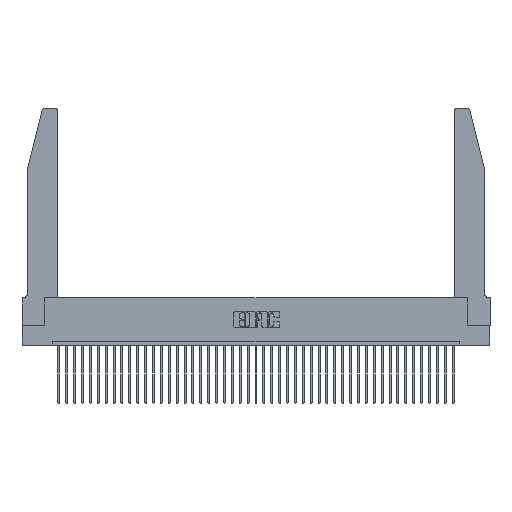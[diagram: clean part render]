
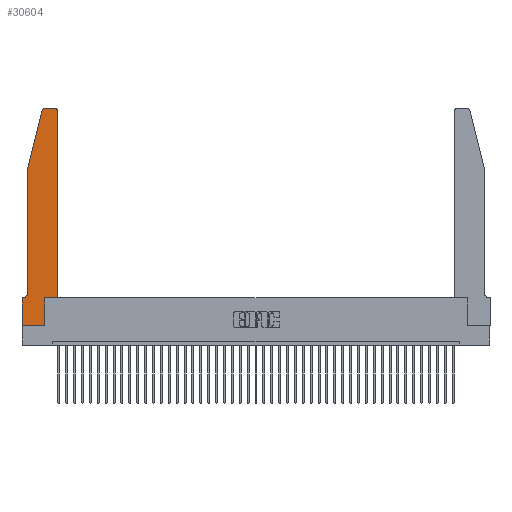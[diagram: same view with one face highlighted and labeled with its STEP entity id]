
A CAD part, top view. The second image highlights one B-rep face of the part: STEP entity #30604.
In plain terms, the highlighted planar face has unit normal (0, 0, 1).
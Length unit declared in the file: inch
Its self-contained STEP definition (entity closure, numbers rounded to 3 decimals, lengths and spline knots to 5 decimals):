
#21 = ORIENTED_EDGE ( 'NONE', *, *, #20833, .T. ) ;
#285 = LINE ( 'NONE', #1883, #33693 ) ;
#905 = AXIS2_PLACEMENT_3D ( 'NONE', #6078, #22050, #25367 ) ;
#1460 = ORIENTED_EDGE ( 'NONE', *, *, #10855, .T. ) ;
#1763 = CARTESIAN_POINT ( 'NONE',  ( 0.0055, 0.35, 0.37 ) ) ;
#1883 = CARTESIAN_POINT ( 'NONE',  ( 0.0755, 2., 0.37 ) ) ;
#2541 = CARTESIAN_POINT ( 'NONE',  ( 0.284, 2.75, 0.37 ) ) ;
#3095 = AXIS2_PLACEMENT_3D ( 'NONE', #4685, #11182, #14152 ) ;
#3257 = LINE ( 'NONE', #5155, #26515 ) ;
#4301 = CARTESIAN_POINT ( 'NONE',  ( 0.2865, 0., 0.37 ) ) ;
#4553 = ORIENTED_EDGE ( 'NONE', *, *, #19292, .T. ) ;
#4685 = CARTESIAN_POINT ( 'NONE',  ( 0., 0.35, 0.37 ) ) ;
#5155 = CARTESIAN_POINT ( 'NONE',  ( 0.0755, 0.35, 0.37 ) ) ;
#5420 = DIRECTION ( 'NONE',  ( 0., -1., 0. ) ) ;
#5426 = ORIENTED_EDGE ( 'NONE', *, *, #34416, .T. ) ;
#5532 = CARTESIAN_POINT ( 'NONE',  ( 0.4505, 2.72, 0.37 ) ) ;
#6078 = CARTESIAN_POINT ( 'NONE',  ( 0.4205, 2.72, 0.37 ) ) ;
#6107 = VERTEX_POINT ( 'NONE', #10280 ) ;
#6631 = AXIS2_PLACEMENT_3D ( 'NONE', #40885, #28096, #11789 ) ;
#6879 = CIRCLE ( 'NONE', #28006, 0.03 ) ;
#7301 = LINE ( 'NONE', #20423, #22028 ) ;
#7570 = LINE ( 'NONE', #35150, #23808 ) ;
#7986 = VERTEX_POINT ( 'NONE', #21831 ) ;
#8224 = VERTEX_POINT ( 'NONE', #38414 ) ;
#8283 = DIRECTION ( 'NONE',  ( 0., 1., 0. ) ) ;
#8423 = FACE_OUTER_BOUND ( 'NONE', #23363, .T. ) ;
#9497 = DIRECTION ( 'NONE',  ( 0., -1., 0. ) ) ;
#10280 = CARTESIAN_POINT ( 'NONE',  ( 0., 0., 0.37 ) ) ;
#10493 = ORIENTED_EDGE ( 'NONE', *, *, #18563, .T. ) ;
#10855 = EDGE_CURVE ( 'NONE', #36951, #17205, #41884, .T. ) ;
#10901 = ORIENTED_EDGE ( 'NONE', *, *, #11124, .T. ) ;
#11124 = EDGE_CURVE ( 'NONE', #15569, #36951, #285, .T. ) ;
#11182 = DIRECTION ( 'NONE',  ( 0., 0., 1. ) ) ;
#11278 = CARTESIAN_POINT ( 'NONE',  ( 0.284, 2.72, 0.37 ) ) ;
#11789 = DIRECTION ( 'NONE',  ( -1., 0., 0. ) ) ;
#12827 = EDGE_CURVE ( 'NONE', #17205, #40345, #3257, .T. ) ;
#12945 = VERTEX_POINT ( 'NONE', #33479 ) ;
#13424 = ORIENTED_EDGE ( 'NONE', *, *, #41559, .T. ) ;
#14152 = DIRECTION ( 'NONE',  ( 1., 0., 0. ) ) ;
#14186 = ORIENTED_EDGE ( 'NONE', *, *, #37096, .T. ) ;
#14284 = CARTESIAN_POINT ( 'NONE',  ( 0.4505, 0.35, 0.37 ) ) ;
#15076 = LINE ( 'NONE', #41703, #27732 ) ;
#15139 = EDGE_CURVE ( 'NONE', #6107, #28270, #30487, .T. ) ;
#15569 = VERTEX_POINT ( 'NONE', #37150 ) ;
#17205 = VERTEX_POINT ( 'NONE', #1763 ) ;
#18095 = CARTESIAN_POINT ( 'NONE',  ( 0.0755, 2., 0.37 ) ) ;
#18563 = EDGE_CURVE ( 'NONE', #39229, #8224, #6879, .T. ) ;
#18691 = LINE ( 'NONE', #18095, #33863 ) ;
#18865 = CARTESIAN_POINT ( 'NONE',  ( 0., 0., 0.37 ) ) ;
#19292 = EDGE_CURVE ( 'NONE', #24825, #26396, #20507, .T. ) ;
#20213 = DIRECTION ( 'NONE',  ( 1., 0., 0. ) ) ;
#20423 = CARTESIAN_POINT ( 'NONE',  ( 0.2865, 0.35, 0.37 ) ) ;
#20507 = LINE ( 'NONE', #41534, #21575 ) ;
#20833 = EDGE_CURVE ( 'NONE', #28270, #7986, #7301, .T. ) ;
#21575 = VECTOR ( 'NONE', #25100, 39.37008 ) ;
#21739 = LINE ( 'NONE', #18865, #41556 ) ;
#21831 = CARTESIAN_POINT ( 'NONE',  ( 0.2865, 0.35, 0.37 ) ) ;
#22028 = VECTOR ( 'NONE', #8283, 39.37008 ) ;
#22050 = DIRECTION ( 'NONE',  ( 0., 0., 1. ) ) ;
#22389 = DIRECTION ( 'NONE',  ( 1., 0., 0. ) ) ;
#22659 = ORIENTED_EDGE ( 'NONE', *, *, #40847, .T. ) ;
#23363 = EDGE_LOOP ( 'NONE', ( #22659, #10493, #5426, #10901, #1460, #26861, #14186, #28476, #21, #33306, #4553, #13424 ) ) ;
#23808 = VECTOR ( 'NONE', #22389, 39.37008 ) ;
#24825 = VERTEX_POINT ( 'NONE', #14284 ) ;
#25100 = DIRECTION ( 'NONE',  ( 0., 1., 0. ) ) ;
#25367 = DIRECTION ( 'NONE',  ( 1., 0., 0. ) ) ;
#25688 = CIRCLE ( 'NONE', #905, 0.03 ) ;
#26396 = VERTEX_POINT ( 'NONE', #5532 ) ;
#26515 = VECTOR ( 'NONE', #40603, 39.37008 ) ;
#26630 = CARTESIAN_POINT ( 'NONE',  ( 0., 0., 0.37 ) ) ;
#26861 = ORIENTED_EDGE ( 'NONE', *, *, #12827, .T. ) ;
#27732 = VECTOR ( 'NONE', #38446, 39.37008 ) ;
#27765 = EDGE_CURVE ( 'NONE', #7986, #24825, #7570, .T. ) ;
#27968 = CARTESIAN_POINT ( 'NONE',  ( 0.0755, 0.42, 0.37 ) ) ;
#28006 = AXIS2_PLACEMENT_3D ( 'NONE', #11278, #33754, #30823 ) ;
#28096 = DIRECTION ( 'NONE',  ( 0., 0., -1. ) ) ;
#28270 = VERTEX_POINT ( 'NONE', #4301 ) ;
#28476 = ORIENTED_EDGE ( 'NONE', *, *, #15139, .T. ) ;
#30487 = LINE ( 'NONE', #26630, #38181 ) ;
#30604 = ADVANCED_FACE ( 'NONE', ( #8423 ), #40249, .T. ) ;
#30823 = DIRECTION ( 'NONE',  ( 1., 0., 0. ) ) ;
#33306 = ORIENTED_EDGE ( 'NONE', *, *, #27765, .T. ) ;
#33479 = CARTESIAN_POINT ( 'NONE',  ( 0.4205, 2.75, 0.37 ) ) ;
#33693 = VECTOR ( 'NONE', #5420, 39.37008 ) ;
#33754 = DIRECTION ( 'NONE',  ( 0., 0., 1. ) ) ;
#33863 = VECTOR ( 'NONE', #34257, 39.37008 ) ;
#34257 = DIRECTION ( 'NONE',  ( -0.239, -0.971, 0. ) ) ;
#34416 = EDGE_CURVE ( 'NONE', #8224, #15569, #18691, .T. ) ;
#35150 = CARTESIAN_POINT ( 'NONE',  ( 0.4505, 0.35, 0.37 ) ) ;
#36951 = VERTEX_POINT ( 'NONE', #27968 ) ;
#37096 = EDGE_CURVE ( 'NONE', #40345, #6107, #21739, .T. ) ;
#37150 = CARTESIAN_POINT ( 'NONE',  ( 0.0755, 2., 0.37 ) ) ;
#37738 = CARTESIAN_POINT ( 'NONE',  ( 0., 0.35, 0.37 ) ) ;
#38181 = VECTOR ( 'NONE', #20213, 39.37008 ) ;
#38414 = CARTESIAN_POINT ( 'NONE',  ( 0.25487, 2.72718, 0.37 ) ) ;
#38446 = DIRECTION ( 'NONE',  ( -1., 0., 0. ) ) ;
#39229 = VERTEX_POINT ( 'NONE', #2541 ) ;
#40249 = PLANE ( 'NONE',  #3095 ) ;
#40345 = VERTEX_POINT ( 'NONE', #37738 ) ;
#40603 = DIRECTION ( 'NONE',  ( -1., 0., 0. ) ) ;
#40847 = EDGE_CURVE ( 'NONE', #12945, #39229, #15076, .T. ) ;
#40885 = CARTESIAN_POINT ( 'NONE',  ( 0.0055, 0.42, 0.37 ) ) ;
#41534 = CARTESIAN_POINT ( 'NONE',  ( 0.4505, 0.35, 0.37 ) ) ;
#41556 = VECTOR ( 'NONE', #9497, 39.37008 ) ;
#41559 = EDGE_CURVE ( 'NONE', #26396, #12945, #25688, .T. ) ;
#41703 = CARTESIAN_POINT ( 'NONE',  ( 0.2605, 2.75, 0.37 ) ) ;
#41884 = CIRCLE ( 'NONE', #6631, 0.07 ) ;
